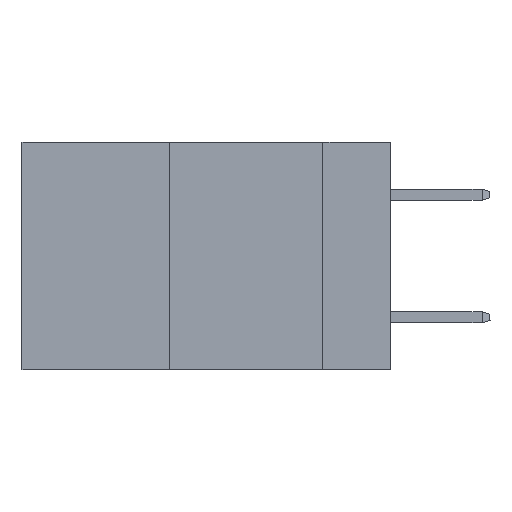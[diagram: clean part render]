
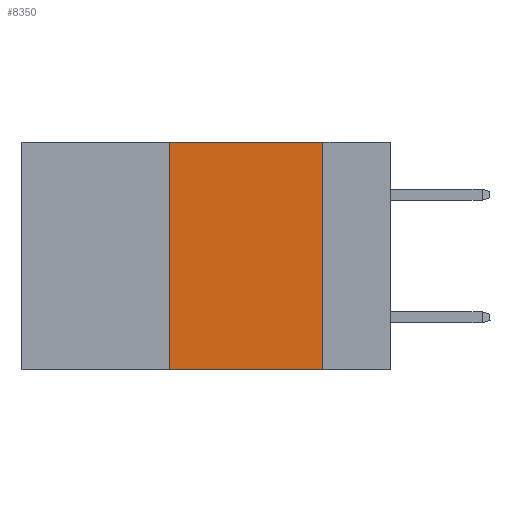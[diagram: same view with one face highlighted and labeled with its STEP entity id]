
A CAD part, left-side view. The second image highlights one B-rep face of the part: STEP entity #8350.
In plain terms, the highlighted planar face has unit normal (-1, 0, 0).
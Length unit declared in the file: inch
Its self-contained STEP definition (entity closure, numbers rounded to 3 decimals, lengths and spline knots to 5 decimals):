
#386 = CARTESIAN_POINT ( 'NONE',  ( 0., 0.11, -0.37 ) ) ;
#922 = DIRECTION ( 'NONE',  ( 0., 0., -1. ) ) ;
#2855 = VECTOR ( 'NONE', #10990, 39.37008 ) ;
#3961 = CARTESIAN_POINT ( 'NONE',  ( 0., 0.36, 0. ) ) ;
#4982 = CARTESIAN_POINT ( 'NONE',  ( 0., 0.36, -0.37 ) ) ;
#6010 = VECTOR ( 'NONE', #7921, 39.37008 ) ;
#6087 = EDGE_LOOP ( 'NONE', ( #21890, #7071, #9210, #12738 ) ) ;
#6233 = DIRECTION ( 'NONE',  ( 0., -1., 0. ) ) ;
#6728 = EDGE_CURVE ( 'NONE', #13135, #11277, #22919, .T. ) ;
#6796 = VERTEX_POINT ( 'NONE', #3961 ) ;
#7071 = ORIENTED_EDGE ( 'NONE', *, *, #22198, .F. ) ;
#7074 = VERTEX_POINT ( 'NONE', #22034 ) ;
#7921 = DIRECTION ( 'NONE',  ( 0., 0., 1. ) ) ;
#8350 = ADVANCED_FACE ( 'NONE', ( #21623 ), #17901, .F. ) ;
#9210 = ORIENTED_EDGE ( 'NONE', *, *, #15120, .F. ) ;
#10018 = DIRECTION ( 'NONE',  ( 0., -1., 0. ) ) ;
#10990 = DIRECTION ( 'NONE',  ( 0., 0., -1. ) ) ;
#11035 = LINE ( 'NONE', #15367, #6010 ) ;
#11277 = VERTEX_POINT ( 'NONE', #386 ) ;
#12252 = DIRECTION ( 'NONE',  ( 1., 0., 0. ) ) ;
#12738 = ORIENTED_EDGE ( 'NONE', *, *, #6728, .T. ) ;
#13084 = LINE ( 'NONE', #23584, #23497 ) ;
#13135 = VERTEX_POINT ( 'NONE', #4982 ) ;
#15120 = EDGE_CURVE ( 'NONE', #13135, #6796, #11035, .T. ) ;
#15306 = CARTESIAN_POINT ( 'NONE',  ( 0., 0.6, -0.37 ) ) ;
#15367 = CARTESIAN_POINT ( 'NONE',  ( 0., 0.36, 0. ) ) ;
#15874 = LINE ( 'NONE', #18215, #2855 ) ;
#16437 = AXIS2_PLACEMENT_3D ( 'NONE', #21723, #12252, #922 ) ;
#17901 = PLANE ( 'NONE',  #16437 ) ;
#18215 = CARTESIAN_POINT ( 'NONE',  ( 0., 0.11, 0. ) ) ;
#20286 = EDGE_CURVE ( 'NONE', #7074, #11277, #15874, .T. ) ;
#20488 = VECTOR ( 'NONE', #10018, 39.37008 ) ;
#21623 = FACE_OUTER_BOUND ( 'NONE', #6087, .T. ) ;
#21723 = CARTESIAN_POINT ( 'NONE',  ( 0., 0.6, 0. ) ) ;
#21890 = ORIENTED_EDGE ( 'NONE', *, *, #20286, .F. ) ;
#22034 = CARTESIAN_POINT ( 'NONE',  ( 0., 0.11, 0. ) ) ;
#22198 = EDGE_CURVE ( 'NONE', #6796, #7074, #13084, .T. ) ;
#22919 = LINE ( 'NONE', #15306, #20488 ) ;
#23497 = VECTOR ( 'NONE', #6233, 39.37008 ) ;
#23584 = CARTESIAN_POINT ( 'NONE',  ( 0., 0.6, 0. ) ) ;
